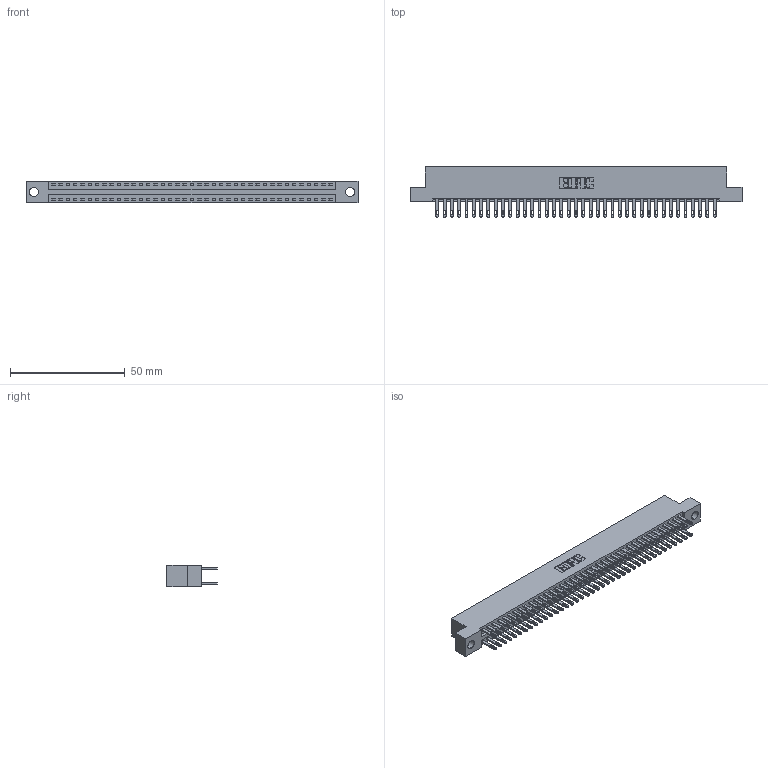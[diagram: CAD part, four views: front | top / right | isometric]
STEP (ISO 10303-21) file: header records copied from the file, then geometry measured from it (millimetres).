
FILE_DESCRIPTION (( 'STEP AP203' ), '1' );
FILE_NAME ('896-078-500-204.STEP', '2021-07-28T01:51:36', ( '' ), ( '' ), 'SwSTEP 2.0', 'SolidWorks 2020', '' );
FILE_SCHEMA (( 'CONFIG_CONTROL_DESIGN' ));
Length unit declared in the file: inch
Products named in the file (3): 345-292-001_345-293-100; 896-078-500-204; 846 Part_Flush Mounting Lugs - 0.156 Dia-TH
Assembly tree (79 placements, depth 2):
  896-078-500-204
    846 Part_Flush Mounting Lugs - 0.156 Dia-TH
    345-292-001_345-293-100  x78
Bounding box: 144.4 x 21.84 x 9.4 mm (x, y, z)
Volume: 14207.9 mm3; surface area: 20112.3 mm2
Topology: 79 solids, 79 shells, 3866 faces, 11795 edges, 7862 vertices
Faces by surface type: plane 2338, cylinder 1528
Entity records: 25789 total; most frequent: CARTESIAN_POINT 4252, ORIENTED_EDGE 4186, DIRECTION 3801, EDGE_CURVE 2093, VECTOR 1801, LINE 1801, VERTEX_POINT 1394, AXIS2_PLACEMENT_3D 1000
